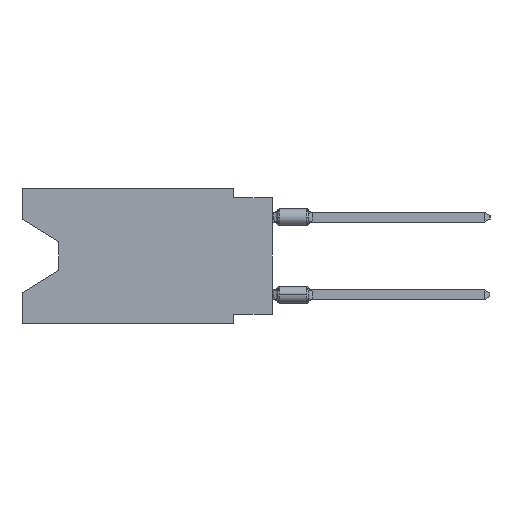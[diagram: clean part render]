
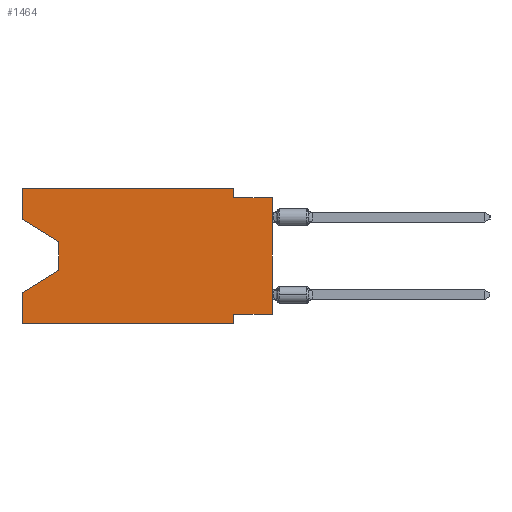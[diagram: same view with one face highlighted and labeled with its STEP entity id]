
A CAD part, left-side view. The second image highlights one B-rep face of the part: STEP entity #1464.
In plain terms, the highlighted planar face has unit normal (-1, 0, 0).
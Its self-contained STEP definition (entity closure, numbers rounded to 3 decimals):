
#237 = DIRECTION ( 'NONE',  ( 0., -1., 0. ) ) ;
#308 = CARTESIAN_POINT ( 'NONE',  ( 0., 0., -8.255 ) ) ;
#330 = CARTESIAN_POINT ( 'NONE',  ( 0., 16.383, -2.038 ) ) ;
#460 = CARTESIAN_POINT ( 'NONE',  ( 0., 16.383, 0. ) ) ;
#790 = ORIENTED_EDGE ( 'NONE', *, *, #5971, .F. ) ;
#794 = VERTEX_POINT ( 'NONE', #3731 ) ;
#1157 = VECTOR ( 'NONE', #22578, 1000. ) ;
#1361 = EDGE_CURVE ( 'NONE', #23363, #10630, #28016, .T. ) ;
#1464 = ADVANCED_FACE ( 'NONE', ( #4933 ), #12006, .F. ) ;
#1518 = EDGE_CURVE ( 'NONE', #20125, #10630, #20151, .T. ) ;
#1743 = VECTOR ( 'NONE', #16407, 1000. ) ;
#1841 = VERTEX_POINT ( 'NONE', #330 ) ;
#2831 = LINE ( 'NONE', #10064, #6302 ) ;
#3712 = VERTEX_POINT ( 'NONE', #24218 ) ;
#3731 = CARTESIAN_POINT ( 'NONE',  ( 0., 13.97, -3.505 ) ) ;
#4033 = VERTEX_POINT ( 'NONE', #460 ) ;
#4129 = CARTESIAN_POINT ( 'NONE',  ( 0., 13.97, -5.385 ) ) ;
#4138 = EDGE_CURVE ( 'NONE', #1841, #794, #2831, .T. ) ;
#4328 = VERTEX_POINT ( 'NONE', #11135 ) ;
#4633 = VECTOR ( 'NONE', #11496, 1000. ) ;
#4710 = VERTEX_POINT ( 'NONE', #12830 ) ;
#4933 = FACE_OUTER_BOUND ( 'NONE', #8621, .T. ) ;
#5100 = ORIENTED_EDGE ( 'NONE', *, *, #23000, .T. ) ;
#5233 = DIRECTION ( 'NONE',  ( 0., 0., -1. ) ) ;
#5482 = VERTEX_POINT ( 'NONE', #29653 ) ;
#5805 = VECTOR ( 'NONE', #237, 1000. ) ;
#5971 = EDGE_CURVE ( 'NONE', #1841, #4033, #20524, .T. ) ;
#6302 = VECTOR ( 'NONE', #27006, 1000. ) ;
#6425 = VECTOR ( 'NONE', #12017, 1000. ) ;
#6472 = ORIENTED_EDGE ( 'NONE', *, *, #15090, .F. ) ;
#6485 = DIRECTION ( 'NONE',  ( 0., 0.855, -0.519 ) ) ;
#6798 = VERTEX_POINT ( 'NONE', #25002 ) ;
#7663 = EDGE_CURVE ( 'NONE', #20125, #6798, #21823, .T. ) ;
#8621 = EDGE_LOOP ( 'NONE', ( #13861, #8818, #9621, #26870, #5100, #10088, #29712, #10342, #19036, #29620, #6472, #790 ) ) ;
#8801 = DIRECTION ( 'NONE',  ( 0., 0., -1. ) ) ;
#8818 = ORIENTED_EDGE ( 'NONE', *, *, #10955, .T. ) ;
#9621 = ORIENTED_EDGE ( 'NONE', *, *, #14176, .T. ) ;
#9855 = VERTEX_POINT ( 'NONE', #17502 ) ;
#10064 = CARTESIAN_POINT ( 'NONE',  ( 0., 16.383, -2.038 ) ) ;
#10070 = VECTOR ( 'NONE', #8801, 1000. ) ;
#10088 = ORIENTED_EDGE ( 'NONE', *, *, #28905, .F. ) ;
#10179 = EDGE_CURVE ( 'NONE', #4710, #5482, #19663, .T. ) ;
#10261 = CARTESIAN_POINT ( 'NONE',  ( 0., 0., 0. ) ) ;
#10342 = ORIENTED_EDGE ( 'NONE', *, *, #1518, .T. ) ;
#10630 = VERTEX_POINT ( 'NONE', #30926 ) ;
#10955 = EDGE_CURVE ( 'NONE', #794, #4328, #16051, .T. ) ;
#11135 = CARTESIAN_POINT ( 'NONE',  ( 0., 13.97, -5.385 ) ) ;
#11173 = CARTESIAN_POINT ( 'NONE',  ( 0., 13.97, -3.505 ) ) ;
#11219 = CARTESIAN_POINT ( 'NONE',  ( 0., 0., -0.635 ) ) ;
#11496 = DIRECTION ( 'NONE',  ( 0., 0., -1. ) ) ;
#11975 = VECTOR ( 'NONE', #20963, 1000. ) ;
#12006 = PLANE ( 'NONE',  #13285 ) ;
#12017 = DIRECTION ( 'NONE',  ( 0., 0., -1. ) ) ;
#12339 = LINE ( 'NONE', #28652, #5805 ) ;
#12830 = CARTESIAN_POINT ( 'NONE',  ( 0., 16.383, -8.89 ) ) ;
#13285 = AXIS2_PLACEMENT_3D ( 'NONE', #16704, #17016, #5233 ) ;
#13861 = ORIENTED_EDGE ( 'NONE', *, *, #4138, .T. ) ;
#14176 = EDGE_CURVE ( 'NONE', #4328, #5482, #27988, .T. ) ;
#14647 = CARTESIAN_POINT ( 'NONE',  ( 0., 16.383, 0. ) ) ;
#15090 = EDGE_CURVE ( 'NONE', #4033, #3712, #30352, .T. ) ;
#15127 = EDGE_CURVE ( 'NONE', #3712, #23363, #19537, .T. ) ;
#15279 = DIRECTION ( 'NONE',  ( 0., 0., 1. ) ) ;
#16051 = LINE ( 'NONE', #11173, #4633 ) ;
#16407 = DIRECTION ( 'NONE',  ( 0., -1., 0. ) ) ;
#16414 = CARTESIAN_POINT ( 'NONE',  ( 0., 2.54, 0. ) ) ;
#16704 = CARTESIAN_POINT ( 'NONE',  ( 0., 16.383, 0. ) ) ;
#17016 = DIRECTION ( 'NONE',  ( 1., 0., 0. ) ) ;
#17502 = CARTESIAN_POINT ( 'NONE',  ( 0., 2.54, -8.89 ) ) ;
#18666 = VECTOR ( 'NONE', #24536, 1000. ) ;
#19036 = ORIENTED_EDGE ( 'NONE', *, *, #1361, .F. ) ;
#19537 = LINE ( 'NONE', #16414, #6425 ) ;
#19663 = LINE ( 'NONE', #14647, #18666 ) ;
#19883 = VECTOR ( 'NONE', #6485, 1000. ) ;
#20125 = VERTEX_POINT ( 'NONE', #28774 ) ;
#20151 = LINE ( 'NONE', #10261, #20741 ) ;
#20524 = LINE ( 'NONE', #29614, #1157 ) ;
#20741 = VECTOR ( 'NONE', #15279, 1000. ) ;
#20786 = CARTESIAN_POINT ( 'NONE',  ( 0., 2.54, -0.635 ) ) ;
#20963 = DIRECTION ( 'NONE',  ( 0., -1., 0. ) ) ;
#21823 = LINE ( 'NONE', #308, #23229 ) ;
#22578 = DIRECTION ( 'NONE',  ( 0., 0., 1. ) ) ;
#23000 = EDGE_CURVE ( 'NONE', #4710, #9855, #12339, .T. ) ;
#23229 = VECTOR ( 'NONE', #23724, 1000. ) ;
#23363 = VERTEX_POINT ( 'NONE', #20786 ) ;
#23386 = CARTESIAN_POINT ( 'NONE',  ( 0., 2.54, -8.89 ) ) ;
#23724 = DIRECTION ( 'NONE',  ( 0., 1., 0. ) ) ;
#24218 = CARTESIAN_POINT ( 'NONE',  ( 0., 2.54, 0. ) ) ;
#24536 = DIRECTION ( 'NONE',  ( 0., 0., 1. ) ) ;
#25002 = CARTESIAN_POINT ( 'NONE',  ( 0., 2.54, -8.255 ) ) ;
#26870 = ORIENTED_EDGE ( 'NONE', *, *, #10179, .F. ) ;
#27006 = DIRECTION ( 'NONE',  ( 0., -0.855, -0.519 ) ) ;
#27988 = LINE ( 'NONE', #4129, #19883 ) ;
#28016 = LINE ( 'NONE', #11219, #1743 ) ;
#28652 = CARTESIAN_POINT ( 'NONE',  ( 0., 16.383, -8.89 ) ) ;
#28774 = CARTESIAN_POINT ( 'NONE',  ( 0., 0., -8.255 ) ) ;
#28905 = EDGE_CURVE ( 'NONE', #6798, #9855, #30731, .T. ) ;
#29614 = CARTESIAN_POINT ( 'NONE',  ( 0., 16.383, 0. ) ) ;
#29620 = ORIENTED_EDGE ( 'NONE', *, *, #15127, .F. ) ;
#29653 = CARTESIAN_POINT ( 'NONE',  ( 0., 16.383, -6.852 ) ) ;
#29712 = ORIENTED_EDGE ( 'NONE', *, *, #7663, .F. ) ;
#30352 = LINE ( 'NONE', #30512, #11975 ) ;
#30512 = CARTESIAN_POINT ( 'NONE',  ( 0., 16.383, 0. ) ) ;
#30731 = LINE ( 'NONE', #23386, #10070 ) ;
#30926 = CARTESIAN_POINT ( 'NONE',  ( 0., 0., -0.635 ) ) ;
